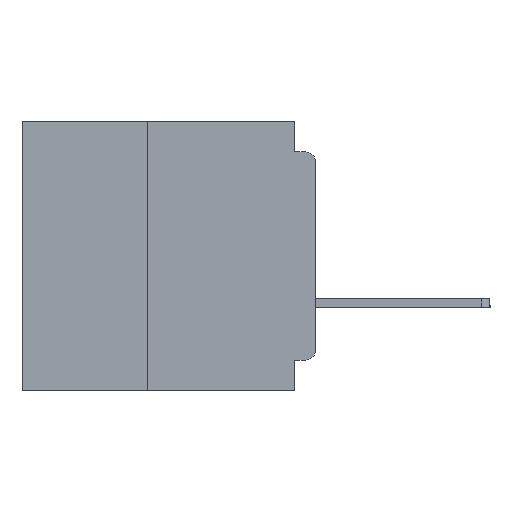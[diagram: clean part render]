
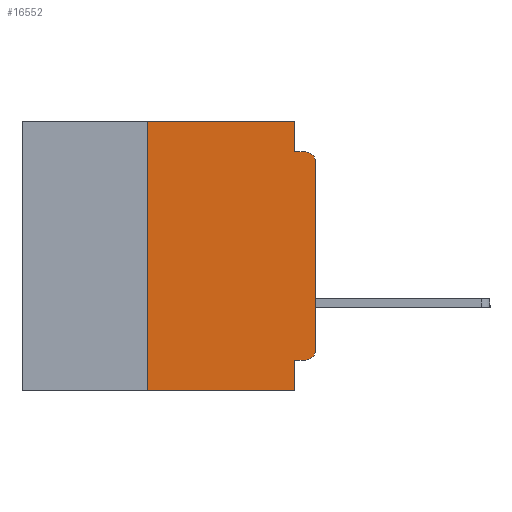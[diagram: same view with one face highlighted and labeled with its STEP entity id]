
A CAD part, left-side view. The second image highlights one B-rep face of the part: STEP entity #16552.
In plain terms, the highlighted planar face has unit normal (-1, 0, 0).
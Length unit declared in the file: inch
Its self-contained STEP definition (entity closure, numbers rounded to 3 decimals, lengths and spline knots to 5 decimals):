
#1672 = ORIENTED_EDGE ( 'NONE', *, *, #4144, .T. ) ;
#1984 = DIRECTION ( 'NONE',  ( 0., 0., 1. ) ) ;
#2639 = DIRECTION ( 'NONE',  ( 0., 0., -1. ) ) ;
#4144 = EDGE_CURVE ( 'NONE', #19956, #47903, #5384, .T. ) ;
#5066 = DIRECTION ( 'NONE',  ( 0., -1., 0. ) ) ;
#5384 = LINE ( 'NONE', #42302, #34017 ) ;
#6376 = CARTESIAN_POINT ( 'NONE',  ( 0., 0., -0.34 ) ) ;
#6437 = CARTESIAN_POINT ( 'NONE',  ( 0., 0.25, 0. ) ) ;
#6447 = DIRECTION ( 'NONE',  ( -1., 0., 0. ) ) ;
#7395 = EDGE_LOOP ( 'NONE', ( #1672, #41865, #20929, #25020, #35477, #18780, #46564, #17463, #32613, #28454 ) ) ;
#8570 = EDGE_CURVE ( 'NONE', #39648, #12414, #30403, .T. ) ;
#8775 = CARTESIAN_POINT ( 'NONE',  ( 0., 0.031, -0.045 ) ) ;
#8798 = CARTESIAN_POINT ( 'NONE',  ( 0., 0.031, 0. ) ) ;
#9424 = VERTEX_POINT ( 'NONE', #12133 ) ;
#9699 = CARTESIAN_POINT ( 'NONE',  ( 0., 0.437, 0. ) ) ;
#10865 = PLANE ( 'NONE',  #20077 ) ;
#11599 = CARTESIAN_POINT ( 'NONE',  ( 0., 0.015, -0.355 ) ) ;
#12133 = CARTESIAN_POINT ( 'NONE',  ( 0., 0.25, -0.4 ) ) ;
#12414 = VERTEX_POINT ( 'NONE', #18383 ) ;
#12840 = EDGE_CURVE ( 'NONE', #42585, #17292, #35290, .T. ) ;
#14496 = DIRECTION ( 'NONE',  ( 0., -1., 0. ) ) ;
#14685 = CIRCLE ( 'NONE', #38392, 0.015 ) ;
#15363 = LINE ( 'NONE', #46294, #35164 ) ;
#16301 = DIRECTION ( 'NONE',  ( 0., 0., 1. ) ) ;
#16552 = ADVANCED_FACE ( 'NONE', ( #21894 ), #10865, .F. ) ;
#17292 = VERTEX_POINT ( 'NONE', #20966 ) ;
#17463 = ORIENTED_EDGE ( 'NONE', *, *, #17708, .F. ) ;
#17708 = EDGE_CURVE ( 'NONE', #43383, #18473, #15363, .T. ) ;
#18096 = VERTEX_POINT ( 'NONE', #11599 ) ;
#18330 = CARTESIAN_POINT ( 'NONE',  ( 0., 0., -0.355 ) ) ;
#18361 = VECTOR ( 'NONE', #44344, 39.37008 ) ;
#18370 = DIRECTION ( 'NONE',  ( 0., 0., -1. ) ) ;
#18383 = CARTESIAN_POINT ( 'NONE',  ( 0., 0.015, -0.045 ) ) ;
#18473 = VERTEX_POINT ( 'NONE', #24769 ) ;
#18780 = ORIENTED_EDGE ( 'NONE', *, *, #20467, .F. ) ;
#19710 = LINE ( 'NONE', #28209, #41844 ) ;
#19956 = VERTEX_POINT ( 'NONE', #6376 ) ;
#19978 = CARTESIAN_POINT ( 'NONE',  ( 0., 0.437, -0.4 ) ) ;
#20077 = AXIS2_PLACEMENT_3D ( 'NONE', #36929, #40688, #18370 ) ;
#20457 = VECTOR ( 'NONE', #34897, 39.37008 ) ;
#20467 = EDGE_CURVE ( 'NONE', #9424, #42585, #19710, .T. ) ;
#20489 = VECTOR ( 'NONE', #14496, 39.37008 ) ;
#20929 = ORIENTED_EDGE ( 'NONE', *, *, #8570, .F. ) ;
#20966 = CARTESIAN_POINT ( 'NONE',  ( 0., 0.031, 0. ) ) ;
#21832 = CARTESIAN_POINT ( 'NONE',  ( 0., 0., -0.045 ) ) ;
#21894 = FACE_OUTER_BOUND ( 'NONE', #7395, .T. ) ;
#22932 = EDGE_CURVE ( 'NONE', #18096, #43383, #48024, .T. ) ;
#24013 = DIRECTION ( 'NONE',  ( 0., 0., -1. ) ) ;
#24402 = VECTOR ( 'NONE', #5066, 39.37008 ) ;
#24516 = DIRECTION ( 'NONE',  ( 0., -1., 0. ) ) ;
#24769 = CARTESIAN_POINT ( 'NONE',  ( 0., 0.031, -0.4 ) ) ;
#25020 = ORIENTED_EDGE ( 'NONE', *, *, #25101, .F. ) ;
#25101 = EDGE_CURVE ( 'NONE', #17292, #39648, #39110, .T. ) ;
#25114 = DIRECTION ( 'NONE',  ( -1., 0., 0. ) ) ;
#25359 = VECTOR ( 'NONE', #24516, 39.37008 ) ;
#28209 = CARTESIAN_POINT ( 'NONE',  ( 0., 0.25, -0.4 ) ) ;
#28454 = ORIENTED_EDGE ( 'NONE', *, *, #37289, .T. ) ;
#28523 = CARTESIAN_POINT ( 'NONE',  ( 0., 0., -0.06 ) ) ;
#28817 = CARTESIAN_POINT ( 'NONE',  ( 0., 0.015, -0.06 ) ) ;
#29506 = EDGE_CURVE ( 'NONE', #9424, #18473, #44173, .T. ) ;
#30403 = LINE ( 'NONE', #21832, #20489 ) ;
#30544 = CARTESIAN_POINT ( 'NONE',  ( 0., 0.031, -0.355 ) ) ;
#32574 = DIRECTION ( 'NONE',  ( 0., 0., -1. ) ) ;
#32613 = ORIENTED_EDGE ( 'NONE', *, *, #22932, .F. ) ;
#34017 = VECTOR ( 'NONE', #16301, 39.37008 ) ;
#34897 = DIRECTION ( 'NONE',  ( 0., 0., -1. ) ) ;
#35164 = VECTOR ( 'NONE', #24013, 39.37008 ) ;
#35290 = LINE ( 'NONE', #9699, #25359 ) ;
#35477 = ORIENTED_EDGE ( 'NONE', *, *, #12840, .F. ) ;
#36929 = CARTESIAN_POINT ( 'NONE',  ( 0., 0.437, 0. ) ) ;
#37289 = EDGE_CURVE ( 'NONE', #18096, #19956, #14685, .T. ) ;
#38237 = AXIS2_PLACEMENT_3D ( 'NONE', #28817, #6447, #32574 ) ;
#38392 = AXIS2_PLACEMENT_3D ( 'NONE', #47367, #25114, #2639 ) ;
#39110 = LINE ( 'NONE', #8798, #20457 ) ;
#39648 = VERTEX_POINT ( 'NONE', #8775 ) ;
#40231 = CIRCLE ( 'NONE', #38237, 0.015 ) ;
#40688 = DIRECTION ( 'NONE',  ( 1., 0., 0. ) ) ;
#41844 = VECTOR ( 'NONE', #1984, 39.37008 ) ;
#41865 = ORIENTED_EDGE ( 'NONE', *, *, #46295, .T. ) ;
#42302 = CARTESIAN_POINT ( 'NONE',  ( 0., 0., 0. ) ) ;
#42585 = VERTEX_POINT ( 'NONE', #6437 ) ;
#43383 = VERTEX_POINT ( 'NONE', #30544 ) ;
#44173 = LINE ( 'NONE', #19978, #24402 ) ;
#44344 = DIRECTION ( 'NONE',  ( 0., 1., 0. ) ) ;
#46294 = CARTESIAN_POINT ( 'NONE',  ( 0., 0.031, -0.4 ) ) ;
#46295 = EDGE_CURVE ( 'NONE', #47903, #12414, #40231, .T. ) ;
#46564 = ORIENTED_EDGE ( 'NONE', *, *, #29506, .T. ) ;
#47367 = CARTESIAN_POINT ( 'NONE',  ( 0., 0.015, -0.34 ) ) ;
#47903 = VERTEX_POINT ( 'NONE', #28523 ) ;
#48024 = LINE ( 'NONE', #18330, #18361 ) ;
